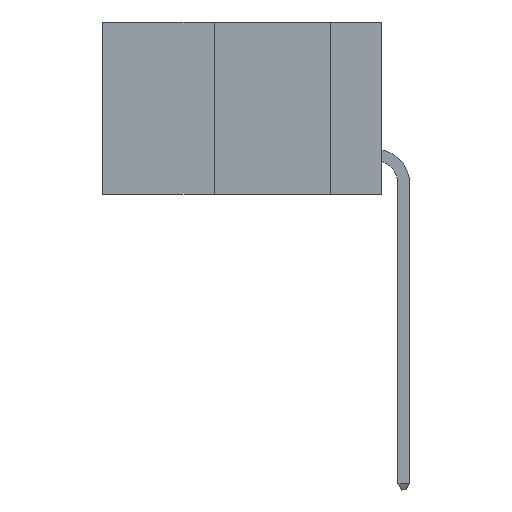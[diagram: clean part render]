
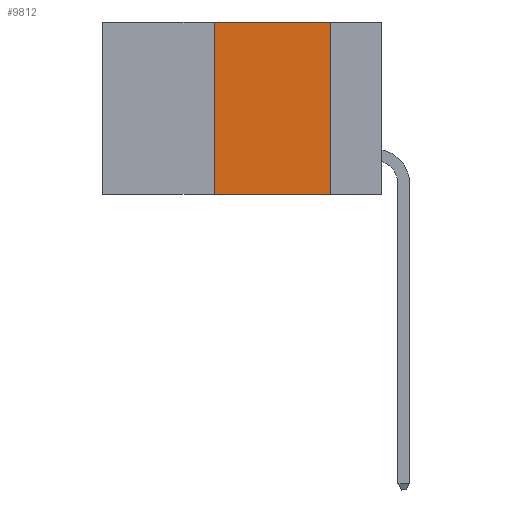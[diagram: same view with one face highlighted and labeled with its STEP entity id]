
A CAD part, left-side view. The second image highlights one B-rep face of the part: STEP entity #9812.
In plain terms, the highlighted planar face has unit normal (-1, 0, 0).
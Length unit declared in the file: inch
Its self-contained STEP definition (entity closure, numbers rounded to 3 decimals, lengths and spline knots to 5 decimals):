
#32 = LINE ( 'NONE', #16116, #19873 ) ;
#1300 = DIRECTION ( 'NONE',  ( 0., 0., -1. ) ) ;
#2042 = FACE_OUTER_BOUND ( 'NONE', #16397, .T. ) ;
#2419 = DIRECTION ( 'NONE',  ( 0., -1., 0. ) ) ;
#2741 = AXIS2_PLACEMENT_3D ( 'NONE', #11589, #4054, #8847 ) ;
#2772 = ORIENTED_EDGE ( 'NONE', *, *, #19875, .F. ) ;
#3010 = EDGE_CURVE ( 'NONE', #15246, #17845, #15340, .T. ) ;
#3481 = DIRECTION ( 'NONE',  ( 0., 0., 1. ) ) ;
#3767 = ORIENTED_EDGE ( 'NONE', *, *, #5349, .F. ) ;
#4054 = DIRECTION ( 'NONE',  ( 1., 0., 0. ) ) ;
#4387 = VECTOR ( 'NONE', #1300, 39.37008 ) ;
#4754 = VECTOR ( 'NONE', #3481, 39.37008 ) ;
#5349 = EDGE_CURVE ( 'NONE', #12580, #17845, #17146, .T. ) ;
#5741 = PLANE ( 'NONE',  #2741 ) ;
#6130 = CARTESIAN_POINT ( 'NONE',  ( 0., 0.11, 0. ) ) ;
#7168 = CARTESIAN_POINT ( 'NONE',  ( 0., 0.11, -0.37 ) ) ;
#7993 = ORIENTED_EDGE ( 'NONE', *, *, #11545, .F. ) ;
#8223 = CARTESIAN_POINT ( 'NONE',  ( 0., 0.36, -0.37 ) ) ;
#8351 = VECTOR ( 'NONE', #18998, 39.37008 ) ;
#8847 = DIRECTION ( 'NONE',  ( 0., 0., -1. ) ) ;
#9530 = LINE ( 'NONE', #10969, #4754 ) ;
#9812 = ADVANCED_FACE ( 'NONE', ( #2042 ), #5741, .F. ) ;
#10579 = CARTESIAN_POINT ( 'NONE',  ( 0., 0.11, 0. ) ) ;
#10969 = CARTESIAN_POINT ( 'NONE',  ( 0., 0.36, 0. ) ) ;
#11545 = EDGE_CURVE ( 'NONE', #12189, #12580, #32, .T. ) ;
#11589 = CARTESIAN_POINT ( 'NONE',  ( 0., 0.6, 0. ) ) ;
#12189 = VERTEX_POINT ( 'NONE', #14566 ) ;
#12580 = VERTEX_POINT ( 'NONE', #6130 ) ;
#14566 = CARTESIAN_POINT ( 'NONE',  ( 0., 0.36, 0. ) ) ;
#15246 = VERTEX_POINT ( 'NONE', #8223 ) ;
#15340 = LINE ( 'NONE', #17507, #8351 ) ;
#16116 = CARTESIAN_POINT ( 'NONE',  ( 0., 0.6, 0. ) ) ;
#16397 = EDGE_LOOP ( 'NONE', ( #3767, #7993, #2772, #17738 ) ) ;
#17146 = LINE ( 'NONE', #10579, #4387 ) ;
#17507 = CARTESIAN_POINT ( 'NONE',  ( 0., 0.6, -0.37 ) ) ;
#17738 = ORIENTED_EDGE ( 'NONE', *, *, #3010, .T. ) ;
#17845 = VERTEX_POINT ( 'NONE', #7168 ) ;
#18998 = DIRECTION ( 'NONE',  ( 0., -1., 0. ) ) ;
#19873 = VECTOR ( 'NONE', #2419, 39.37008 ) ;
#19875 = EDGE_CURVE ( 'NONE', #15246, #12189, #9530, .T. ) ;
